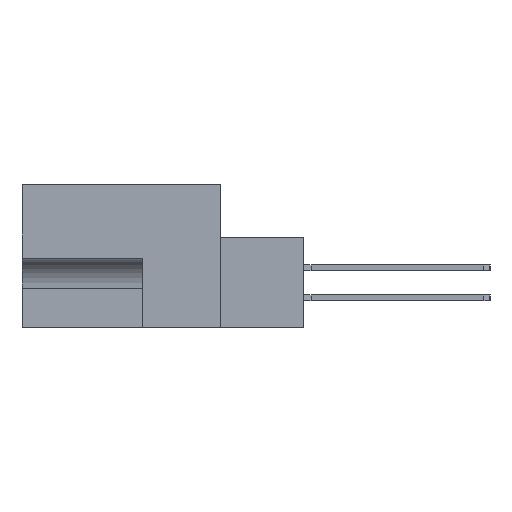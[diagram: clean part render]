
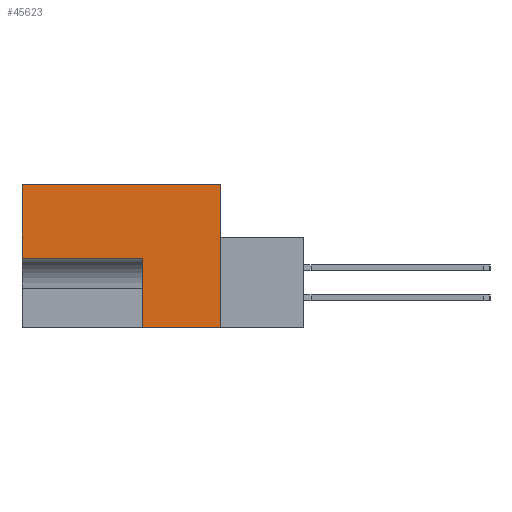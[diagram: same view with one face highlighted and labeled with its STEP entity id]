
A CAD part, left-side view. The second image highlights one B-rep face of the part: STEP entity #45623.
In plain terms, the highlighted planar face has unit normal (-1, 0, 0).
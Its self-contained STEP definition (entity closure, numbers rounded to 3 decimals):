
#98 = FACE_OUTER_BOUND ( 'NONE', #48890, .T. ) ;
#456 = CARTESIAN_POINT ( 'NONE',  ( 0., 20.955, 0. ) ) ;
#1000 = VECTOR ( 'NONE', #5443, 1000. ) ;
#1856 = VECTOR ( 'NONE', #51626, 1000. ) ;
#2336 = DIRECTION ( 'NONE',  ( 0., -1., 0. ) ) ;
#2481 = CARTESIAN_POINT ( 'NONE',  ( 0., 20.955, -7.772 ) ) ;
#3108 = CARTESIAN_POINT ( 'NONE',  ( 0., 8.255, -7.772 ) ) ;
#4009 = VERTEX_POINT ( 'NONE', #2481 ) ;
#4934 = CARTESIAN_POINT ( 'NONE',  ( 0., -8.814, -15.088 ) ) ;
#5443 = DIRECTION ( 'NONE',  ( 0., 1., 0. ) ) ;
#7748 = VERTEX_POINT ( 'NONE', #3108 ) ;
#9241 = ORIENTED_EDGE ( 'NONE', *, *, #31311, .F. ) ;
#9334 = VECTOR ( 'NONE', #25239, 1000. ) ;
#12099 = CARTESIAN_POINT ( 'NONE',  ( 0., 0., 0. ) ) ;
#14225 = LINE ( 'NONE', #4934, #1000 ) ;
#15116 = LINE ( 'NONE', #36318, #18857 ) ;
#15462 = PLANE ( 'NONE',  #24079 ) ;
#18857 = VECTOR ( 'NONE', #48218, 1000. ) ;
#19605 = ORIENTED_EDGE ( 'NONE', *, *, #49222, .F. ) ;
#21249 = CARTESIAN_POINT ( 'NONE',  ( 0., 0., -15.088 ) ) ;
#23976 = DIRECTION ( 'NONE',  ( 1., 0., 0. ) ) ;
#24079 = AXIS2_PLACEMENT_3D ( 'NONE', #47414, #23976, #27458 ) ;
#25239 = DIRECTION ( 'NONE',  ( 0., 0., -1. ) ) ;
#25942 = VECTOR ( 'NONE', #50327, 1000. ) ;
#27458 = DIRECTION ( 'NONE',  ( 0., 0., -1. ) ) ;
#27652 = VERTEX_POINT ( 'NONE', #38069 ) ;
#29668 = ORIENTED_EDGE ( 'NONE', *, *, #41560, .F. ) ;
#30619 = VERTEX_POINT ( 'NONE', #456 ) ;
#30943 = LINE ( 'NONE', #45619, #25942 ) ;
#31311 = EDGE_CURVE ( 'NONE', #49036, #27652, #14225, .T. ) ;
#35645 = LINE ( 'NONE', #39238, #1856 ) ;
#36318 = CARTESIAN_POINT ( 'NONE',  ( 0., 20.955, -15.088 ) ) ;
#36937 = EDGE_CURVE ( 'NONE', #43020, #49036, #43734, .T. ) ;
#38069 = CARTESIAN_POINT ( 'NONE',  ( 0., 8.255, -15.088 ) ) ;
#38608 = VECTOR ( 'NONE', #2336, 1000. ) ;
#38703 = CARTESIAN_POINT ( 'NONE',  ( 0., 11.506, 0. ) ) ;
#39237 = ORIENTED_EDGE ( 'NONE', *, *, #39566, .F. ) ;
#39238 = CARTESIAN_POINT ( 'NONE',  ( 0., 8.255, -15.088 ) ) ;
#39566 = EDGE_CURVE ( 'NONE', #7748, #4009, #30943, .T. ) ;
#39856 = LINE ( 'NONE', #38703, #38608 ) ;
#40946 = CARTESIAN_POINT ( 'NONE',  ( 0., 0., 0. ) ) ;
#41560 = EDGE_CURVE ( 'NONE', #4009, #30619, #15116, .T. ) ;
#42137 = EDGE_CURVE ( 'NONE', #27652, #7748, #35645, .T. ) ;
#43020 = VERTEX_POINT ( 'NONE', #12099 ) ;
#43393 = ORIENTED_EDGE ( 'NONE', *, *, #42137, .F. ) ;
#43734 = LINE ( 'NONE', #40946, #9334 ) ;
#45619 = CARTESIAN_POINT ( 'NONE',  ( 0., 8.255, -7.772 ) ) ;
#45623 = ADVANCED_FACE ( 'NONE', ( #98 ), #15462, .F. ) ;
#47414 = CARTESIAN_POINT ( 'NONE',  ( 0., 0., 0. ) ) ;
#47597 = ORIENTED_EDGE ( 'NONE', *, *, #36937, .F. ) ;
#48218 = DIRECTION ( 'NONE',  ( 0., 0., 1. ) ) ;
#48890 = EDGE_LOOP ( 'NONE', ( #9241, #47597, #19605, #29668, #39237, #43393 ) ) ;
#49036 = VERTEX_POINT ( 'NONE', #21249 ) ;
#49222 = EDGE_CURVE ( 'NONE', #30619, #43020, #39856, .T. ) ;
#50327 = DIRECTION ( 'NONE',  ( 0., 1., 0. ) ) ;
#51626 = DIRECTION ( 'NONE',  ( 0., 0., 1. ) ) ;
